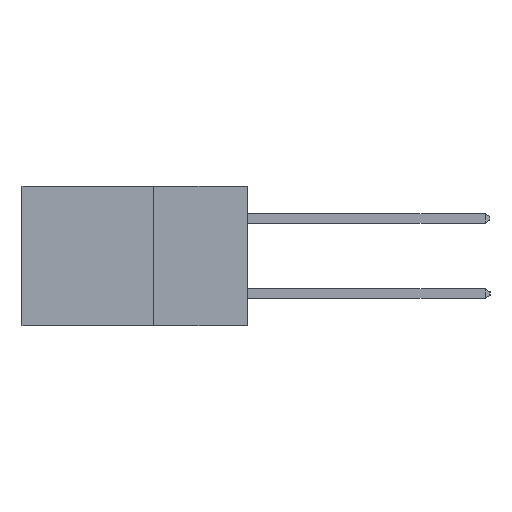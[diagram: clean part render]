
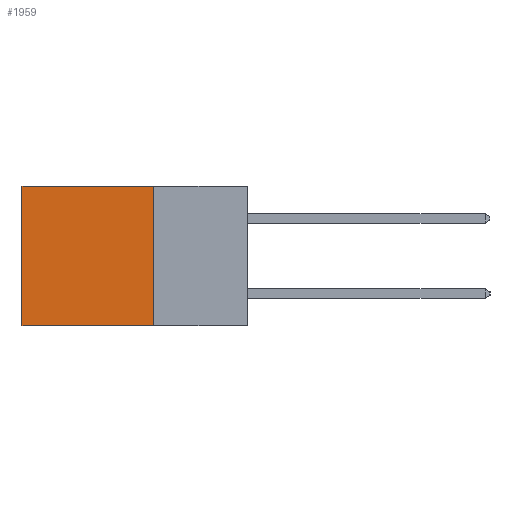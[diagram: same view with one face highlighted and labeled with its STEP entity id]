
A CAD part, left-side view. The second image highlights one B-rep face of the part: STEP entity #1959.
In plain terms, the highlighted planar face has unit normal (-1, 0, 0).
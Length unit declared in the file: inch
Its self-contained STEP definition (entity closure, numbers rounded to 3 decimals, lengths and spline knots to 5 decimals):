
#1957 = CARTESIAN_POINT ( 'NONE',  ( 0.2615, 0.25, 0. ) ) ;
#1959 = ADVANCED_FACE ( 'NONE', ( #2968 ), #6680, .F. ) ;
#2800 = VECTOR ( 'NONE', #4815, 39.37008 ) ;
#2934 = DIRECTION ( 'NONE',  ( 0., 1., 0. ) ) ;
#2945 = CARTESIAN_POINT ( 'NONE',  ( 0.2615, 0.25, -0.37 ) ) ;
#2968 = FACE_OUTER_BOUND ( 'NONE', #5957, .T. ) ;
#3114 = CARTESIAN_POINT ( 'NONE',  ( 0.2615, 0.25, -0.37 ) ) ;
#3725 = DIRECTION ( 'NONE',  ( 0., 1., 0. ) ) ;
#3856 = CARTESIAN_POINT ( 'NONE',  ( 0.2615, 0.25, 0. ) ) ;
#3877 = VERTEX_POINT ( 'NONE', #6265 ) ;
#4312 = DIRECTION ( 'NONE',  ( 0., 0., -1. ) ) ;
#4321 = VECTOR ( 'NONE', #2934, 39.37008 ) ;
#4435 = VECTOR ( 'NONE', #10169, 39.37008 ) ;
#4815 = DIRECTION ( 'NONE',  ( 0., 0., -1. ) ) ;
#4861 = CARTESIAN_POINT ( 'NONE',  ( 0.2615, 0.6, -0.37 ) ) ;
#5579 = CARTESIAN_POINT ( 'NONE',  ( 0.2615, 0.25, -0.37 ) ) ;
#5957 = EDGE_LOOP ( 'NONE', ( #6087, #7600, #6866, #6740 ) ) ;
#6087 = ORIENTED_EDGE ( 'NONE', *, *, #6245, .T. ) ;
#6117 = VECTOR ( 'NONE', #3725, 39.37008 ) ;
#6245 = EDGE_CURVE ( 'NONE', #3877, #8610, #7795, .T. ) ;
#6265 = CARTESIAN_POINT ( 'NONE',  ( 0.2615, 0.6, 0. ) ) ;
#6680 = PLANE ( 'NONE',  #11182 ) ;
#6740 = ORIENTED_EDGE ( 'NONE', *, *, #9897, .T. ) ;
#6756 = CARTESIAN_POINT ( 'NONE',  ( 0.2615, 0.25, -0.37 ) ) ;
#6851 = LINE ( 'NONE', #3114, #4321 ) ;
#6866 = ORIENTED_EDGE ( 'NONE', *, *, #10783, .F. ) ;
#6984 = LINE ( 'NONE', #5579, #4435 ) ;
#7600 = ORIENTED_EDGE ( 'NONE', *, *, #10044, .F. ) ;
#7795 = LINE ( 'NONE', #4861, #2800 ) ;
#8247 = CARTESIAN_POINT ( 'NONE',  ( 0.2615, 0.6, -0.37 ) ) ;
#8610 = VERTEX_POINT ( 'NONE', #8247 ) ;
#9897 = EDGE_CURVE ( 'NONE', #11526, #3877, #11266, .T. ) ;
#10044 = EDGE_CURVE ( 'NONE', #10067, #8610, #6851, .T. ) ;
#10067 = VERTEX_POINT ( 'NONE', #2945 ) ;
#10169 = DIRECTION ( 'NONE',  ( 0., 0., -1. ) ) ;
#10783 = EDGE_CURVE ( 'NONE', #11526, #10067, #6984, .T. ) ;
#11182 = AXIS2_PLACEMENT_3D ( 'NONE', #6756, #11570, #4312 ) ;
#11266 = LINE ( 'NONE', #3856, #6117 ) ;
#11526 = VERTEX_POINT ( 'NONE', #1957 ) ;
#11570 = DIRECTION ( 'NONE',  ( 1., 0., 0. ) ) ;
